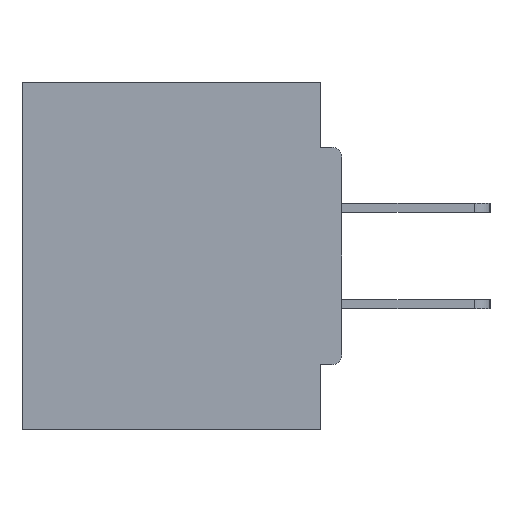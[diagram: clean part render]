
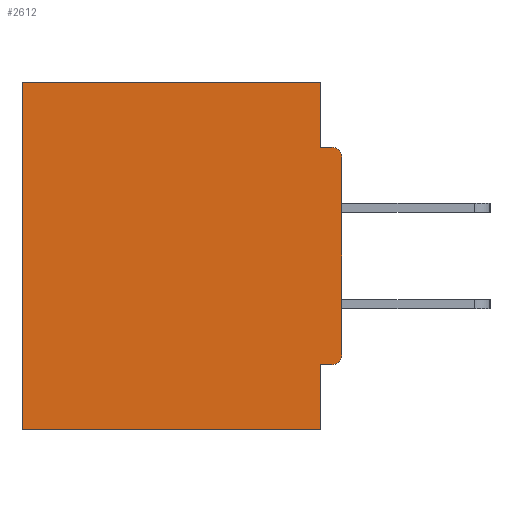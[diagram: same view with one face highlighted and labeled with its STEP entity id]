
A CAD part, left-side view. The second image highlights one B-rep face of the part: STEP entity #2612.
In plain terms, the highlighted planar face has unit normal (-1, 0, 0).
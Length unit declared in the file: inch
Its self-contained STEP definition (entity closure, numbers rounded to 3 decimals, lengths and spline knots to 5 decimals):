
#263 = AXIS2_PLACEMENT_3D ( 'NONE', #7111, #30145, #24774 ) ;
#757 = ORIENTED_EDGE ( 'NONE', *, *, #9511, .F. ) ;
#1632 = CARTESIAN_POINT ( 'NONE',  ( 0.298, 0.46, 0. ) ) ;
#1759 = DIRECTION ( 'NONE',  ( 0., 0., -1. ) ) ;
#2003 = LINE ( 'NONE', #20287, #17004 ) ;
#2374 = CARTESIAN_POINT ( 'NONE',  ( 0.298, 0.015, -0.0935 ) ) ;
#2566 = VERTEX_POINT ( 'NONE', #12048 ) ;
#2612 = ADVANCED_FACE ( 'NONE', ( #12120 ), #14893, .F. ) ;
#3109 = CARTESIAN_POINT ( 'NONE',  ( 0.298, 0.46, -0.5 ) ) ;
#4019 = LINE ( 'NONE', #20874, #26077 ) ;
#4079 = CIRCLE ( 'NONE', #26761, 0.015 ) ;
#4146 = ORIENTED_EDGE ( 'NONE', *, *, #22458, .F. ) ;
#5219 = ORIENTED_EDGE ( 'NONE', *, *, #12637, .T. ) ;
#5237 = VECTOR ( 'NONE', #14668, 39.37008 ) ;
#5851 = CARTESIAN_POINT ( 'NONE',  ( 0.298, 0.031, -0.0935 ) ) ;
#6758 = VERTEX_POINT ( 'NONE', #1632 ) ;
#7107 = CARTESIAN_POINT ( 'NONE',  ( 0.298, 0.031, -0.5 ) ) ;
#7111 = CARTESIAN_POINT ( 'NONE',  ( 0.298, 0., 0. ) ) ;
#7676 = EDGE_LOOP ( 'NONE', ( #15719, #22167, #21649, #5219, #25364, #757, #20831, #4146, #14261, #14572 ) ) ;
#8164 = VECTOR ( 'NONE', #24696, 39.37008 ) ;
#8383 = DIRECTION ( 'NONE',  ( 0., 1., 0. ) ) ;
#8922 = AXIS2_PLACEMENT_3D ( 'NONE', #16858, #11811, #1759 ) ;
#9140 = CARTESIAN_POINT ( 'NONE',  ( 0.298, 0.031, -0.5 ) ) ;
#9328 = LINE ( 'NONE', #9140, #25844 ) ;
#9511 = EDGE_CURVE ( 'NONE', #26241, #25908, #14811, .T. ) ;
#9845 = VECTOR ( 'NONE', #16742, 39.37008 ) ;
#9906 = CARTESIAN_POINT ( 'NONE',  ( 0.298, 0.031, 0. ) ) ;
#9978 = LINE ( 'NONE', #24105, #24943 ) ;
#10136 = CARTESIAN_POINT ( 'NONE',  ( 0.298, 0.015, -0.1085 ) ) ;
#11670 = VERTEX_POINT ( 'NONE', #9906 ) ;
#11705 = EDGE_CURVE ( 'NONE', #19261, #30833, #4079, .T. ) ;
#11811 = DIRECTION ( 'NONE',  ( -1., 0., 0. ) ) ;
#12048 = CARTESIAN_POINT ( 'NONE',  ( 0.298, 0.015, -0.4065 ) ) ;
#12120 = FACE_OUTER_BOUND ( 'NONE', #7676, .T. ) ;
#12604 = CARTESIAN_POINT ( 'NONE',  ( 0.298, 0., -0.1085 ) ) ;
#12637 = EDGE_CURVE ( 'NONE', #11670, #6758, #4019, .T. ) ;
#12717 = EDGE_CURVE ( 'NONE', #6758, #25908, #2003, .T. ) ;
#12921 = EDGE_CURVE ( 'NONE', #19261, #28470, #27603, .T. ) ;
#13797 = CARTESIAN_POINT ( 'NONE',  ( 0.298, 0., 0. ) ) ;
#14261 = ORIENTED_EDGE ( 'NONE', *, *, #23581, .T. ) ;
#14572 = ORIENTED_EDGE ( 'NONE', *, *, #12921, .F. ) ;
#14668 = DIRECTION ( 'NONE',  ( 0., -1., 0. ) ) ;
#14811 = LINE ( 'NONE', #18668, #8164 ) ;
#14893 = PLANE ( 'NONE',  #263 ) ;
#15719 = ORIENTED_EDGE ( 'NONE', *, *, #11705, .T. ) ;
#16742 = DIRECTION ( 'NONE',  ( 0., 0., -1. ) ) ;
#16858 = CARTESIAN_POINT ( 'NONE',  ( 0.298, 0.015, -0.3915 ) ) ;
#17004 = VECTOR ( 'NONE', #32559, 39.37008 ) ;
#18178 = CARTESIAN_POINT ( 'NONE',  ( 0.298, 0.031, -0.5 ) ) ;
#18668 = CARTESIAN_POINT ( 'NONE',  ( 0.298, 0., -0.5 ) ) ;
#18774 = EDGE_CURVE ( 'NONE', #11670, #32052, #32579, .T. ) ;
#19261 = VERTEX_POINT ( 'NONE', #12604 ) ;
#19707 = CARTESIAN_POINT ( 'NONE',  ( 0.298, 0., -0.0935 ) ) ;
#20005 = DIRECTION ( 'NONE',  ( 0., 0., -1. ) ) ;
#20287 = CARTESIAN_POINT ( 'NONE',  ( 0.298, 0.46, 0. ) ) ;
#20524 = CIRCLE ( 'NONE', #8922, 0.015 ) ;
#20831 = ORIENTED_EDGE ( 'NONE', *, *, #24110, .F. ) ;
#20874 = CARTESIAN_POINT ( 'NONE',  ( 0.298, 0., 0. ) ) ;
#21649 = ORIENTED_EDGE ( 'NONE', *, *, #18774, .F. ) ;
#22167 = ORIENTED_EDGE ( 'NONE', *, *, #26155, .F. ) ;
#22458 = EDGE_CURVE ( 'NONE', #2566, #26613, #9978, .T. ) ;
#23581 = EDGE_CURVE ( 'NONE', #2566, #28470, #20524, .T. ) ;
#24105 = CARTESIAN_POINT ( 'NONE',  ( 0.298, 0., -0.4065 ) ) ;
#24110 = EDGE_CURVE ( 'NONE', #26613, #26241, #9328, .T. ) ;
#24696 = DIRECTION ( 'NONE',  ( 0., 1., 0. ) ) ;
#24774 = DIRECTION ( 'NONE',  ( 0., 0., -1. ) ) ;
#24838 = DIRECTION ( 'NONE',  ( -1., 0., 0. ) ) ;
#24943 = VECTOR ( 'NONE', #32397, 39.37008 ) ;
#25364 = ORIENTED_EDGE ( 'NONE', *, *, #12717, .T. ) ;
#25844 = VECTOR ( 'NONE', #26712, 39.37008 ) ;
#25908 = VERTEX_POINT ( 'NONE', #3109 ) ;
#26077 = VECTOR ( 'NONE', #8383, 39.37008 ) ;
#26155 = EDGE_CURVE ( 'NONE', #32052, #30833, #28432, .T. ) ;
#26241 = VERTEX_POINT ( 'NONE', #7107 ) ;
#26428 = CARTESIAN_POINT ( 'NONE',  ( 0.298, 0.031, -0.4065 ) ) ;
#26452 = VECTOR ( 'NONE', #28851, 39.37008 ) ;
#26613 = VERTEX_POINT ( 'NONE', #26428 ) ;
#26712 = DIRECTION ( 'NONE',  ( 0., 0., -1. ) ) ;
#26761 = AXIS2_PLACEMENT_3D ( 'NONE', #10136, #24838, #20005 ) ;
#27603 = LINE ( 'NONE', #13797, #26452 ) ;
#28432 = LINE ( 'NONE', #19707, #5237 ) ;
#28470 = VERTEX_POINT ( 'NONE', #30024 ) ;
#28851 = DIRECTION ( 'NONE',  ( 0., 0., -1. ) ) ;
#30024 = CARTESIAN_POINT ( 'NONE',  ( 0.298, 0., -0.3915 ) ) ;
#30145 = DIRECTION ( 'NONE',  ( 1., 0., 0. ) ) ;
#30833 = VERTEX_POINT ( 'NONE', #2374 ) ;
#32052 = VERTEX_POINT ( 'NONE', #5851 ) ;
#32397 = DIRECTION ( 'NONE',  ( 0., 1., 0. ) ) ;
#32559 = DIRECTION ( 'NONE',  ( 0., 0., -1. ) ) ;
#32579 = LINE ( 'NONE', #18178, #9845 ) ;
